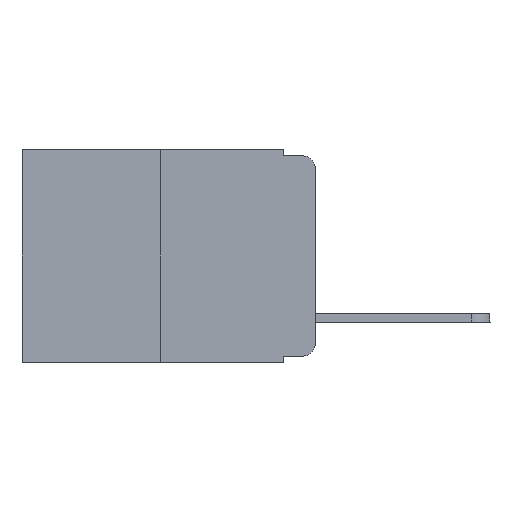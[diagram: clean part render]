
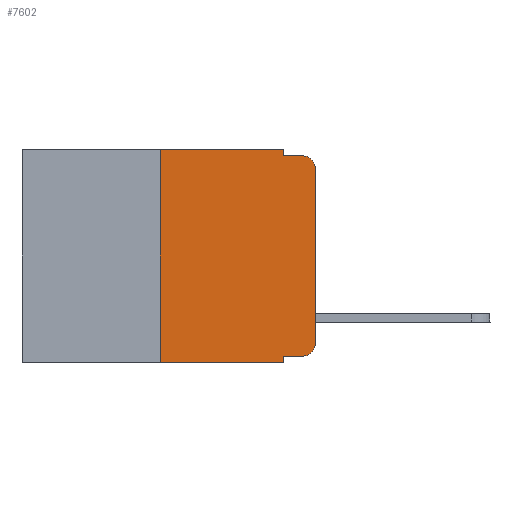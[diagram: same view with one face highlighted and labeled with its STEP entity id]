
A CAD part, left-side view. The second image highlights one B-rep face of the part: STEP entity #7602.
In plain terms, the highlighted planar face has unit normal (-1, 0, 0).
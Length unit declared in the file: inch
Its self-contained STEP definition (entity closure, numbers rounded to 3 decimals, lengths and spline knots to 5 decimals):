
#14 = VECTOR ( 'NONE', #16612, 39.37008 ) ;
#20 = EDGE_CURVE ( 'NONE', #2527, #3684, #15359, .T. ) ;
#108 = DIRECTION ( 'NONE',  ( 1., 0., 0. ) ) ;
#282 = VERTEX_POINT ( 'NONE', #12522 ) ;
#556 = CARTESIAN_POINT ( 'NONE',  ( 0., 0.02, -0.01 ) ) ;
#652 = VECTOR ( 'NONE', #6896, 39.37008 ) ;
#717 = DIRECTION ( 'NONE',  ( 0., 0., 1. ) ) ;
#737 = ORIENTED_EDGE ( 'NONE', *, *, #5402, .F. ) ;
#769 = VERTEX_POINT ( 'NONE', #1645 ) ;
#965 = CARTESIAN_POINT ( 'NONE',  ( 0., 0.051, -0.01 ) ) ;
#1325 = VECTOR ( 'NONE', #6879, 39.37008 ) ;
#1468 = EDGE_CURVE ( 'NONE', #2527, #8318, #16300, .T. ) ;
#1494 = ORIENTED_EDGE ( 'NONE', *, *, #1468, .F. ) ;
#1645 = CARTESIAN_POINT ( 'NONE',  ( 0., 0.051, 0. ) ) ;
#1865 = CARTESIAN_POINT ( 'NONE',  ( 0., 0.051, 0. ) ) ;
#2135 = ORIENTED_EDGE ( 'NONE', *, *, #4995, .F. ) ;
#2189 = VERTEX_POINT ( 'NONE', #6105 ) ;
#2286 = LINE ( 'NONE', #10079, #14 ) ;
#2527 = VERTEX_POINT ( 'NONE', #14569 ) ;
#2573 = ORIENTED_EDGE ( 'NONE', *, *, #5271, .T. ) ;
#2719 = ORIENTED_EDGE ( 'NONE', *, *, #8645, .T. ) ;
#2865 = LINE ( 'NONE', #8623, #5498 ) ;
#2938 = CARTESIAN_POINT ( 'NONE',  ( 0., 0.25, 0. ) ) ;
#3053 = DIRECTION ( 'NONE',  ( 0., 0., -1. ) ) ;
#3133 = EDGE_CURVE ( 'NONE', #16506, #769, #8696, .T. ) ;
#3403 = DIRECTION ( 'NONE',  ( 0., -1., 0. ) ) ;
#3413 = DIRECTION ( 'NONE',  ( 0., -1., 0. ) ) ;
#3684 = VERTEX_POINT ( 'NONE', #12306 ) ;
#4012 = DIRECTION ( 'NONE',  ( 0., 0., -1. ) ) ;
#4138 = DIRECTION ( 'NONE',  ( -1., 0., 0. ) ) ;
#4351 = CARTESIAN_POINT ( 'NONE',  ( 0., 0.051, -0.343 ) ) ;
#4802 = DIRECTION ( 'NONE',  ( 0., -1., 0. ) ) ;
#4995 = EDGE_CURVE ( 'NONE', #769, #8848, #2286, .T. ) ;
#5228 = CIRCLE ( 'NONE', #14842, 0.02 ) ;
#5271 = EDGE_CURVE ( 'NONE', #3684, #282, #15099, .T. ) ;
#5402 = EDGE_CURVE ( 'NONE', #8848, #8785, #2865, .T. ) ;
#5498 = VECTOR ( 'NONE', #3403, 39.37008 ) ;
#5514 = ORIENTED_EDGE ( 'NONE', *, *, #3133, .F. ) ;
#5787 = ORIENTED_EDGE ( 'NONE', *, *, #11518, .T. ) ;
#5997 = VECTOR ( 'NONE', #4802, 39.37008 ) ;
#6105 = CARTESIAN_POINT ( 'NONE',  ( 0., 0., -0.03 ) ) ;
#6618 = VECTOR ( 'NONE', #717, 39.37008 ) ;
#6761 = CARTESIAN_POINT ( 'NONE',  ( 0., 0.473, 0. ) ) ;
#6879 = DIRECTION ( 'NONE',  ( 0., 0., 1. ) ) ;
#6896 = DIRECTION ( 'NONE',  ( 0., -1., 0. ) ) ;
#6898 = CARTESIAN_POINT ( 'NONE',  ( 0., 0.02, -0.313 ) ) ;
#6996 = CARTESIAN_POINT ( 'NONE',  ( 0., 0., 0. ) ) ;
#7518 = ORIENTED_EDGE ( 'NONE', *, *, #8890, .T. ) ;
#7572 = CARTESIAN_POINT ( 'NONE',  ( 0., 0.473, -0.343 ) ) ;
#7602 = ADVANCED_FACE ( 'NONE', ( #9334 ), #10771, .F. ) ;
#7683 = AXIS2_PLACEMENT_3D ( 'NONE', #6898, #4138, #13208 ) ;
#8118 = CARTESIAN_POINT ( 'NONE',  ( 0., 0.473, 0. ) ) ;
#8318 = VERTEX_POINT ( 'NONE', #4351 ) ;
#8623 = CARTESIAN_POINT ( 'NONE',  ( 0., 0.051, -0.01 ) ) ;
#8645 = EDGE_CURVE ( 'NONE', #282, #2189, #9084, .T. ) ;
#8696 = LINE ( 'NONE', #8118, #9508 ) ;
#8785 = VERTEX_POINT ( 'NONE', #556 ) ;
#8848 = VERTEX_POINT ( 'NONE', #965 ) ;
#8890 = EDGE_CURVE ( 'NONE', #12607, #8318, #15969, .T. ) ;
#9084 = LINE ( 'NONE', #6996, #1325 ) ;
#9334 = FACE_OUTER_BOUND ( 'NONE', #12085, .T. ) ;
#9455 = ORIENTED_EDGE ( 'NONE', *, *, #11881, .F. ) ;
#9508 = VECTOR ( 'NONE', #3413, 39.37008 ) ;
#10079 = CARTESIAN_POINT ( 'NONE',  ( 0., 0.051, 0. ) ) ;
#10459 = CARTESIAN_POINT ( 'NONE',  ( 0., 0.02, -0.03 ) ) ;
#10620 = DIRECTION ( 'NONE',  ( 0., 0., -1. ) ) ;
#10771 = PLANE ( 'NONE',  #13864 ) ;
#10932 = CARTESIAN_POINT ( 'NONE',  ( 0., 0.25, 0. ) ) ;
#11518 = EDGE_CURVE ( 'NONE', #2189, #8785, #5228, .T. ) ;
#11881 = EDGE_CURVE ( 'NONE', #12607, #16506, #14005, .T. ) ;
#12085 = EDGE_LOOP ( 'NONE', ( #2719, #5787, #737, #2135, #5514, #9455, #7518, #1494, #12765, #2573 ) ) ;
#12306 = CARTESIAN_POINT ( 'NONE',  ( 0., 0.02, -0.333 ) ) ;
#12522 = CARTESIAN_POINT ( 'NONE',  ( 0., 0., -0.313 ) ) ;
#12607 = VERTEX_POINT ( 'NONE', #12927 ) ;
#12765 = ORIENTED_EDGE ( 'NONE', *, *, #20, .T. ) ;
#12927 = CARTESIAN_POINT ( 'NONE',  ( 0., 0.25, -0.343 ) ) ;
#13208 = DIRECTION ( 'NONE',  ( 0., 0., -1. ) ) ;
#13864 = AXIS2_PLACEMENT_3D ( 'NONE', #6761, #108, #4012 ) ;
#14005 = LINE ( 'NONE', #10932, #6618 ) ;
#14442 = DIRECTION ( 'NONE',  ( -1., 0., 0. ) ) ;
#14569 = CARTESIAN_POINT ( 'NONE',  ( 0., 0.051, -0.333 ) ) ;
#14769 = CARTESIAN_POINT ( 'NONE',  ( 0., 0.051, -0.333 ) ) ;
#14842 = AXIS2_PLACEMENT_3D ( 'NONE', #10459, #14442, #10620 ) ;
#15099 = CIRCLE ( 'NONE', #7683, 0.02 ) ;
#15359 = LINE ( 'NONE', #14769, #652 ) ;
#15969 = LINE ( 'NONE', #7572, #5997 ) ;
#16300 = LINE ( 'NONE', #1865, #16505 ) ;
#16505 = VECTOR ( 'NONE', #3053, 39.37008 ) ;
#16506 = VERTEX_POINT ( 'NONE', #2938 ) ;
#16612 = DIRECTION ( 'NONE',  ( 0., 0., -1. ) ) ;
